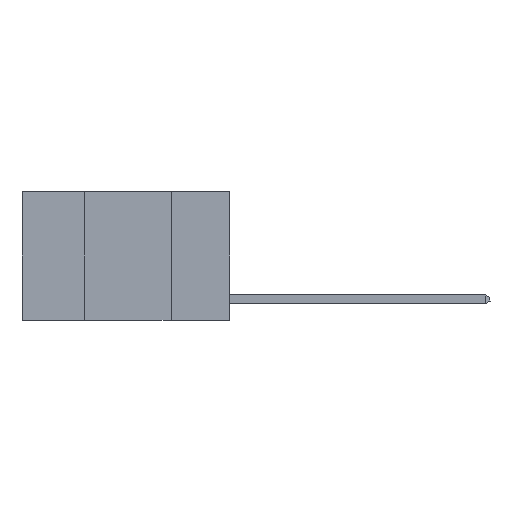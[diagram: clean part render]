
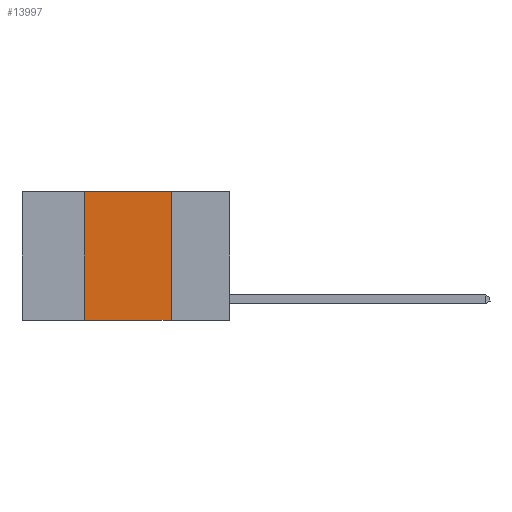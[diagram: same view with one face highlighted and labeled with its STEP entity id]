
A CAD part, left-side view. The second image highlights one B-rep face of the part: STEP entity #13997.
In plain terms, the highlighted planar face has unit normal (-1, 0, 0).
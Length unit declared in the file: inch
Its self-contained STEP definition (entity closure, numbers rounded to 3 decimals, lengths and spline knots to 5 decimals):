
#792 = LINE ( 'NONE', #2145, #9724 ) ;
#909 = CARTESIAN_POINT ( 'NONE',  ( 0., 0.17, 0. ) ) ;
#1269 = DIRECTION ( 'NONE',  ( 0., 0., 1. ) ) ;
#2145 = CARTESIAN_POINT ( 'NONE',  ( 0., 0.6, 0. ) ) ;
#2165 = ORIENTED_EDGE ( 'NONE', *, *, #8125, .F. ) ;
#2739 = ORIENTED_EDGE ( 'NONE', *, *, #5744, .T. ) ;
#2747 = DIRECTION ( 'NONE',  ( 0., 0., -1. ) ) ;
#3532 = CARTESIAN_POINT ( 'NONE',  ( 0., 0.6, 0. ) ) ;
#3836 = LINE ( 'NONE', #11845, #4251 ) ;
#3991 = DIRECTION ( 'NONE',  ( 0., -1., 0. ) ) ;
#4251 = VECTOR ( 'NONE', #22326, 39.37008 ) ;
#5744 = EDGE_CURVE ( 'NONE', #22238, #12128, #3836, .T. ) ;
#5801 = AXIS2_PLACEMENT_3D ( 'NONE', #3532, #19346, #8884 ) ;
#6922 = EDGE_CURVE ( 'NONE', #22238, #19695, #8102, .T. ) ;
#7227 = EDGE_CURVE ( 'NONE', #19695, #16102, #792, .T. ) ;
#8102 = LINE ( 'NONE', #22360, #16886 ) ;
#8125 = EDGE_CURVE ( 'NONE', #16102, #12128, #19512, .T. ) ;
#8884 = DIRECTION ( 'NONE',  ( 0., 0., -1. ) ) ;
#9724 = VECTOR ( 'NONE', #3991, 39.37008 ) ;
#10230 = VECTOR ( 'NONE', #2747, 39.37008 ) ;
#11618 = ORIENTED_EDGE ( 'NONE', *, *, #7227, .F. ) ;
#11845 = CARTESIAN_POINT ( 'NONE',  ( 0., 0.6, -0.37 ) ) ;
#12128 = VERTEX_POINT ( 'NONE', #14248 ) ;
#13997 = ADVANCED_FACE ( 'NONE', ( #14084 ), #22752, .F. ) ;
#14084 = FACE_OUTER_BOUND ( 'NONE', #19830, .T. ) ;
#14248 = CARTESIAN_POINT ( 'NONE',  ( 0., 0.17, -0.37 ) ) ;
#15283 = CARTESIAN_POINT ( 'NONE',  ( 0., 0.17, 0. ) ) ;
#16102 = VERTEX_POINT ( 'NONE', #15283 ) ;
#16886 = VECTOR ( 'NONE', #1269, 39.37008 ) ;
#19322 = CARTESIAN_POINT ( 'NONE',  ( 0., 0.42, -0.37 ) ) ;
#19346 = DIRECTION ( 'NONE',  ( 1., 0., 0. ) ) ;
#19512 = LINE ( 'NONE', #909, #10230 ) ;
#19695 = VERTEX_POINT ( 'NONE', #21372 ) ;
#19830 = EDGE_LOOP ( 'NONE', ( #2165, #11618, #20888, #2739 ) ) ;
#20888 = ORIENTED_EDGE ( 'NONE', *, *, #6922, .F. ) ;
#21372 = CARTESIAN_POINT ( 'NONE',  ( 0., 0.42, 0. ) ) ;
#22238 = VERTEX_POINT ( 'NONE', #19322 ) ;
#22326 = DIRECTION ( 'NONE',  ( 0., -1., 0. ) ) ;
#22360 = CARTESIAN_POINT ( 'NONE',  ( 0., 0.42, 0. ) ) ;
#22752 = PLANE ( 'NONE',  #5801 ) ;
